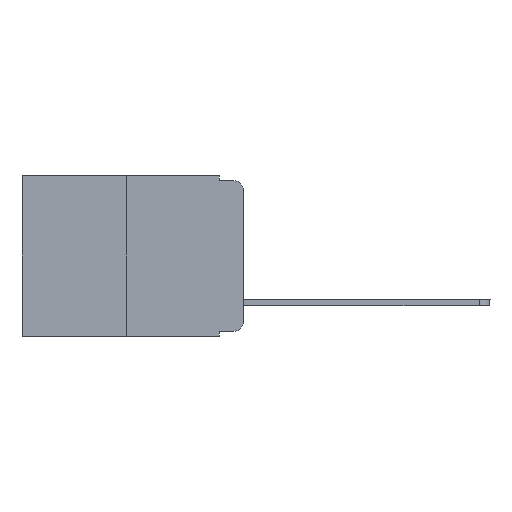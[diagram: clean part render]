
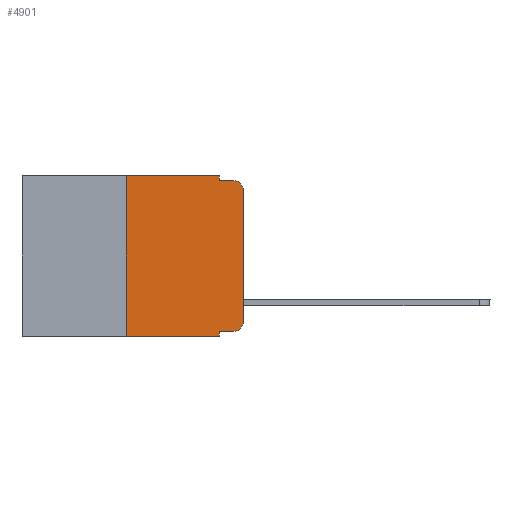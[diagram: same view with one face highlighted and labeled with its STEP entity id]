
A CAD part, left-side view. The second image highlights one B-rep face of the part: STEP entity #4901.
In plain terms, the highlighted planar face has unit normal (-1, 0, 0).
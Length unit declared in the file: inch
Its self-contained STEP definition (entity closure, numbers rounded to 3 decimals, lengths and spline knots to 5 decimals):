
#315 = AXIS2_PLACEMENT_3D ( 'NONE', #6275, #1835, #1605 ) ;
#477 = CARTESIAN_POINT ( 'NONE',  ( 0., 0.051, 0. ) ) ;
#618 = EDGE_CURVE ( 'NONE', #13754, #9518, #3671, .T. ) ;
#623 = VERTEX_POINT ( 'NONE', #2817 ) ;
#900 = CARTESIAN_POINT ( 'NONE',  ( 0., 0.051, 0. ) ) ;
#965 = DIRECTION ( 'NONE',  ( 1., 0., 0. ) ) ;
#1044 = PLANE ( 'NONE',  #8415 ) ;
#1193 = CARTESIAN_POINT ( 'NONE',  ( 0., 0.473, 0. ) ) ;
#1204 = AXIS2_PLACEMENT_3D ( 'NONE', #9542, #1678, #14244 ) ;
#1605 = DIRECTION ( 'NONE',  ( 0., 0., -1. ) ) ;
#1678 = DIRECTION ( 'NONE',  ( -1., 0., 0. ) ) ;
#1694 = VECTOR ( 'NONE', #5661, 39.37008 ) ;
#1835 = DIRECTION ( 'NONE',  ( -1., 0., 0. ) ) ;
#2240 = CARTESIAN_POINT ( 'NONE',  ( 0., 0.473, 0. ) ) ;
#2688 = LINE ( 'NONE', #477, #7490 ) ;
#2817 = CARTESIAN_POINT ( 'NONE',  ( 0., 0.051, -0.01 ) ) ;
#3000 = CARTESIAN_POINT ( 'NONE',  ( 0., 0., -0.313 ) ) ;
#3018 = EDGE_LOOP ( 'NONE', ( #8729, #10994, #11740, #3489, #8684, #7545, #11118, #3610, #11467, #14209 ) ) ;
#3027 = DIRECTION ( 'NONE',  ( 0., -1., 0. ) ) ;
#3383 = EDGE_CURVE ( 'NONE', #3624, #623, #7032, .T. ) ;
#3489 = ORIENTED_EDGE ( 'NONE', *, *, #3383, .F. ) ;
#3610 = ORIENTED_EDGE ( 'NONE', *, *, #7925, .F. ) ;
#3624 = VERTEX_POINT ( 'NONE', #7003 ) ;
#3671 = CIRCLE ( 'NONE', #315, 0.02 ) ;
#3955 = VERTEX_POINT ( 'NONE', #14931 ) ;
#4159 = CARTESIAN_POINT ( 'NONE',  ( 0., 0.25, 0. ) ) ;
#4262 = VERTEX_POINT ( 'NONE', #14912 ) ;
#4541 = EDGE_CURVE ( 'NONE', #9518, #13509, #11618, .T. ) ;
#4901 = ADVANCED_FACE ( 'NONE', ( #13992 ), #1044, .F. ) ;
#5399 = VECTOR ( 'NONE', #8876, 39.37008 ) ;
#5661 = DIRECTION ( 'NONE',  ( 0., -1., 0. ) ) ;
#5732 = CARTESIAN_POINT ( 'NONE',  ( 0., 0.02, -0.333 ) ) ;
#5796 = CARTESIAN_POINT ( 'NONE',  ( 0., 0., 0. ) ) ;
#5853 = DIRECTION ( 'NONE',  ( 0., 0., -1. ) ) ;
#6275 = CARTESIAN_POINT ( 'NONE',  ( 0., 0.02, -0.313 ) ) ;
#6305 = DIRECTION ( 'NONE',  ( 0., 0., -1. ) ) ;
#6487 = CARTESIAN_POINT ( 'NONE',  ( 0., 0.051, -0.333 ) ) ;
#6510 = VECTOR ( 'NONE', #9337, 39.37008 ) ;
#6613 = CIRCLE ( 'NONE', #1204, 0.02 ) ;
#6656 = CARTESIAN_POINT ( 'NONE',  ( 0., 0.051, -0.343 ) ) ;
#7003 = CARTESIAN_POINT ( 'NONE',  ( 0., 0.051, 0. ) ) ;
#7032 = LINE ( 'NONE', #900, #14504 ) ;
#7490 = VECTOR ( 'NONE', #6305, 39.37008 ) ;
#7545 = ORIENTED_EDGE ( 'NONE', *, *, #13210, .F. ) ;
#7576 = EDGE_CURVE ( 'NONE', #3955, #13754, #14748, .T. ) ;
#7586 = EDGE_CURVE ( 'NONE', #623, #10967, #12310, .T. ) ;
#7858 = EDGE_CURVE ( 'NONE', #12971, #3624, #13891, .T. ) ;
#7925 = EDGE_CURVE ( 'NONE', #3955, #10400, #2688, .T. ) ;
#8415 = AXIS2_PLACEMENT_3D ( 'NONE', #1193, #965, #5853 ) ;
#8684 = ORIENTED_EDGE ( 'NONE', *, *, #7858, .F. ) ;
#8729 = ORIENTED_EDGE ( 'NONE', *, *, #4541, .T. ) ;
#8876 = DIRECTION ( 'NONE',  ( 0., 0., 1. ) ) ;
#9191 = VECTOR ( 'NONE', #14672, 39.37008 ) ;
#9337 = DIRECTION ( 'NONE',  ( 0., -1., 0. ) ) ;
#9518 = VERTEX_POINT ( 'NONE', #3000 ) ;
#9542 = CARTESIAN_POINT ( 'NONE',  ( 0., 0.02, -0.03 ) ) ;
#10327 = CARTESIAN_POINT ( 'NONE',  ( 0., 0.02, -0.01 ) ) ;
#10400 = VERTEX_POINT ( 'NONE', #6656 ) ;
#10454 = DIRECTION ( 'NONE',  ( 0., 0., 1. ) ) ;
#10967 = VERTEX_POINT ( 'NONE', #10327 ) ;
#10994 = ORIENTED_EDGE ( 'NONE', *, *, #11551, .T. ) ;
#11114 = LINE ( 'NONE', #4159, #5399 ) ;
#11118 = ORIENTED_EDGE ( 'NONE', *, *, #11311, .T. ) ;
#11311 = EDGE_CURVE ( 'NONE', #4262, #10400, #13860, .T. ) ;
#11467 = ORIENTED_EDGE ( 'NONE', *, *, #7576, .T. ) ;
#11551 = EDGE_CURVE ( 'NONE', #13509, #10967, #6613, .T. ) ;
#11618 = LINE ( 'NONE', #5796, #14529 ) ;
#11687 = DIRECTION ( 'NONE',  ( 0., 0., -1. ) ) ;
#11740 = ORIENTED_EDGE ( 'NONE', *, *, #7586, .F. ) ;
#12035 = CARTESIAN_POINT ( 'NONE',  ( 0., 0., -0.03 ) ) ;
#12310 = LINE ( 'NONE', #13531, #12880 ) ;
#12684 = CARTESIAN_POINT ( 'NONE',  ( 0., 0.25, 0. ) ) ;
#12880 = VECTOR ( 'NONE', #3027, 39.37008 ) ;
#12933 = CARTESIAN_POINT ( 'NONE',  ( 0., 0.473, -0.343 ) ) ;
#12971 = VERTEX_POINT ( 'NONE', #12684 ) ;
#13210 = EDGE_CURVE ( 'NONE', #4262, #12971, #11114, .T. ) ;
#13509 = VERTEX_POINT ( 'NONE', #12035 ) ;
#13531 = CARTESIAN_POINT ( 'NONE',  ( 0., 0.051, -0.01 ) ) ;
#13754 = VERTEX_POINT ( 'NONE', #5732 ) ;
#13860 = LINE ( 'NONE', #12933, #1694 ) ;
#13891 = LINE ( 'NONE', #2240, #6510 ) ;
#13992 = FACE_OUTER_BOUND ( 'NONE', #3018, .T. ) ;
#14209 = ORIENTED_EDGE ( 'NONE', *, *, #618, .T. ) ;
#14244 = DIRECTION ( 'NONE',  ( 0., 0., -1. ) ) ;
#14504 = VECTOR ( 'NONE', #11687, 39.37008 ) ;
#14529 = VECTOR ( 'NONE', #10454, 39.37008 ) ;
#14672 = DIRECTION ( 'NONE',  ( 0., -1., 0. ) ) ;
#14748 = LINE ( 'NONE', #6487, #9191 ) ;
#14912 = CARTESIAN_POINT ( 'NONE',  ( 0., 0.25, -0.343 ) ) ;
#14931 = CARTESIAN_POINT ( 'NONE',  ( 0., 0.051, -0.333 ) ) ;
